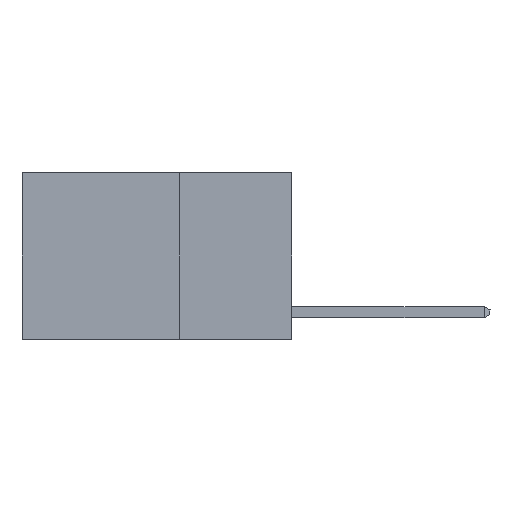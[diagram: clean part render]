
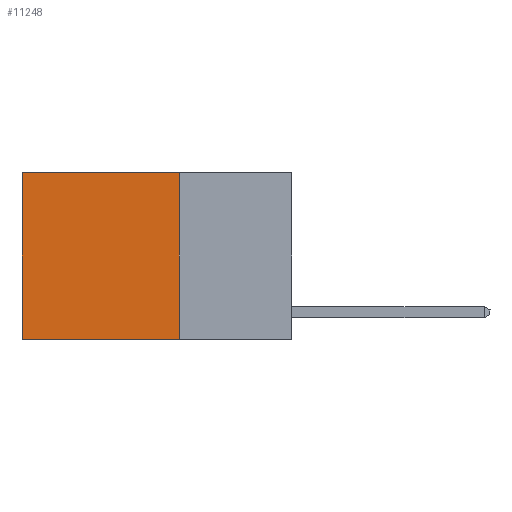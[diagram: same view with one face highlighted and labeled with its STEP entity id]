
A CAD part, left-side view. The second image highlights one B-rep face of the part: STEP entity #11248.
In plain terms, the highlighted planar face has unit normal (-1, 0, 0).
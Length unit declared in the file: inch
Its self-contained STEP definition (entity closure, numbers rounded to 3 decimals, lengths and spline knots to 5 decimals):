
#309 = ORIENTED_EDGE ( 'NONE', *, *, #14674, .T. ) ;
#755 = EDGE_CURVE ( 'NONE', #2137, #2874, #11623, .T. ) ;
#1163 = VECTOR ( 'NONE', #13151, 39.37008 ) ;
#1712 = ORIENTED_EDGE ( 'NONE', *, *, #2864, .F. ) ;
#1817 = EDGE_LOOP ( 'NONE', ( #309, #1712, #8029, #10627 ) ) ;
#2137 = VERTEX_POINT ( 'NONE', #5301 ) ;
#2344 = AXIS2_PLACEMENT_3D ( 'NONE', #11781, #15773, #7815 ) ;
#2864 = EDGE_CURVE ( 'NONE', #16694, #16435, #4442, .T. ) ;
#2874 = VERTEX_POINT ( 'NONE', #7059 ) ;
#3298 = EDGE_CURVE ( 'NONE', #2137, #16694, #11550, .T. ) ;
#3862 = CARTESIAN_POINT ( 'NONE',  ( 0.2625, 0.25, -0.37 ) ) ;
#4442 = LINE ( 'NONE', #7661, #7586 ) ;
#4652 = CARTESIAN_POINT ( 'NONE',  ( 0.2625, 0.6, -0.37 ) ) ;
#5301 = CARTESIAN_POINT ( 'NONE',  ( 0.2625, 0.25, 0. ) ) ;
#5335 = FACE_OUTER_BOUND ( 'NONE', #1817, .T. ) ;
#6566 = LINE ( 'NONE', #13158, #17083 ) ;
#7059 = CARTESIAN_POINT ( 'NONE',  ( 0.2625, 0.6, 0. ) ) ;
#7586 = VECTOR ( 'NONE', #8168, 39.37008 ) ;
#7651 = VECTOR ( 'NONE', #15370, 39.37008 ) ;
#7661 = CARTESIAN_POINT ( 'NONE',  ( 0.2625, 0.25, -0.37 ) ) ;
#7815 = DIRECTION ( 'NONE',  ( 0., 0., -1. ) ) ;
#8029 = ORIENTED_EDGE ( 'NONE', *, *, #3298, .F. ) ;
#8168 = DIRECTION ( 'NONE',  ( 0., 1., 0. ) ) ;
#9174 = DIRECTION ( 'NONE',  ( 0., 0., -1. ) ) ;
#10173 = CARTESIAN_POINT ( 'NONE',  ( 0.2625, 0.25, 0. ) ) ;
#10627 = ORIENTED_EDGE ( 'NONE', *, *, #755, .T. ) ;
#11248 = ADVANCED_FACE ( 'NONE', ( #5335 ), #14477, .F. ) ;
#11550 = LINE ( 'NONE', #13105, #1163 ) ;
#11623 = LINE ( 'NONE', #10173, #7651 ) ;
#11781 = CARTESIAN_POINT ( 'NONE',  ( 0.2625, 0.25, 0. ) ) ;
#13105 = CARTESIAN_POINT ( 'NONE',  ( 0.2625, 0.25, 0. ) ) ;
#13151 = DIRECTION ( 'NONE',  ( 0., 0., -1. ) ) ;
#13158 = CARTESIAN_POINT ( 'NONE',  ( 0.2625, 0.6, 0. ) ) ;
#14477 = PLANE ( 'NONE',  #2344 ) ;
#14674 = EDGE_CURVE ( 'NONE', #2874, #16435, #6566, .T. ) ;
#15370 = DIRECTION ( 'NONE',  ( 0., 1., 0. ) ) ;
#15773 = DIRECTION ( 'NONE',  ( 1., 0., 0. ) ) ;
#16435 = VERTEX_POINT ( 'NONE', #4652 ) ;
#16694 = VERTEX_POINT ( 'NONE', #3862 ) ;
#17083 = VECTOR ( 'NONE', #9174, 39.37008 ) ;
